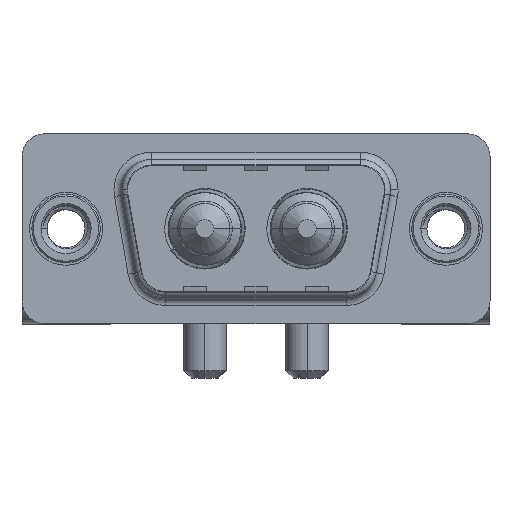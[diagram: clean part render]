
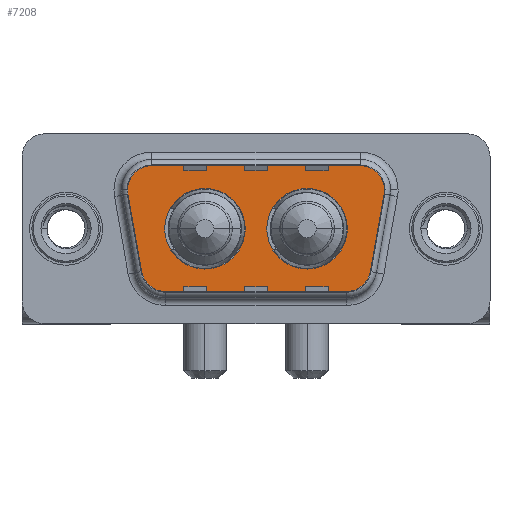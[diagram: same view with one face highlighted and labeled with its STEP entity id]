
A CAD part, top view. The second image highlights one B-rep face of the part: STEP entity #7208.
In plain terms, the highlighted planar face has unit normal (0, 0, 1).
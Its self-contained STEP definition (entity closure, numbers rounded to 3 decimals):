
#143 = CARTESIAN_POINT ( 'NONE',  ( 11.79, 0., 0. ) ) ;
#180 = VERTEX_POINT ( 'NONE', #11453 ) ;
#261 = CARTESIAN_POINT ( 'NONE',  ( 19.564, 2.9, 0. ) ) ;
#269 = EDGE_CURVE ( 'NONE', #180, #8889, #14029, .T. ) ;
#319 = EDGE_CURVE ( 'NONE', #8889, #8603, #11657, .T. ) ;
#706 = DIRECTION ( 'NONE',  ( 0., 0., 1. ) ) ;
#756 = CIRCLE ( 'NONE', #9415, 2. ) ;
#801 = CIRCLE ( 'NONE', #8774, 2.65 ) ;
#992 = CARTESIAN_POINT ( 'NONE',  ( 4.489, -3.247, 0. ) ) ;
#1006 = EDGE_CURVE ( 'NONE', #6856, #180, #7688, .T. ) ;
#1249 = CIRCLE ( 'NONE', #12812, 2.65 ) ;
#1399 = ORIENTED_EDGE ( 'NONE', *, *, #6689, .T. ) ;
#1654 = DIRECTION ( 'NONE',  ( -1., 0., 0. ) ) ;
#1833 = CARTESIAN_POINT ( 'NONE',  ( 3.466, 2.553, 0. ) ) ;
#1867 = DIRECTION ( 'NONE',  ( 0., 0., 1. ) ) ;
#1878 = CARTESIAN_POINT ( 'NONE',  ( 9.14, 0., 0. ) ) ;
#1929 = CARTESIAN_POINT ( 'NONE',  ( 21.534, 2.553, 0. ) ) ;
#1938 = CARTESIAN_POINT ( 'NONE',  ( 3.466, 2.553, 0. ) ) ;
#1943 = AXIS2_PLACEMENT_3D ( 'NONE', #5372, #4238, #2030 ) ;
#1968 = VERTEX_POINT ( 'NONE', #12082 ) ;
#2030 = DIRECTION ( 'NONE',  ( -1., 0., 0. ) ) ;
#2038 = CARTESIAN_POINT ( 'NONE',  ( 6.459, -4.9, 0. ) ) ;
#2361 = FACE_BOUND ( 'NONE', #6490, .T. ) ;
#2383 = AXIS2_PLACEMENT_3D ( 'NONE', #10458, #706, #2593 ) ;
#2424 = CARTESIAN_POINT ( 'NONE',  ( 5.436, 4.9, 0. ) ) ;
#2593 = DIRECTION ( 'NONE',  ( 1., 0., 0. ) ) ;
#2623 = CIRCLE ( 'NONE', #2383, 2.65 ) ;
#2870 = CARTESIAN_POINT ( 'NONE',  ( 6.459, -2.9, 0. ) ) ;
#3503 = CIRCLE ( 'NONE', #10978, 2. ) ;
#3579 = ORIENTED_EDGE ( 'NONE', *, *, #5162, .F. ) ;
#3752 = VERTEX_POINT ( 'NONE', #8855 ) ;
#4012 = EDGE_CURVE ( 'NONE', #6295, #6856, #756, .T. ) ;
#4131 = CARTESIAN_POINT ( 'NONE',  ( 20.511, -3.247, 0. ) ) ;
#4238 = DIRECTION ( 'NONE',  ( 0., 0., 1. ) ) ;
#4376 = CARTESIAN_POINT ( 'NONE',  ( 15.86, 0., 0. ) ) ;
#4553 = DIRECTION ( 'NONE',  ( -1., 0., 0. ) ) ;
#4625 = DIRECTION ( 'NONE',  ( 0., 0., 1. ) ) ;
#4734 = ORIENTED_EDGE ( 'NONE', *, *, #7578, .T. ) ;
#4845 = DIRECTION ( 'NONE',  ( 1., 0., 0. ) ) ;
#4931 = VERTEX_POINT ( 'NONE', #143 ) ;
#4943 = DIRECTION ( 'NONE',  ( 1., 0., 0. ) ) ;
#4959 = EDGE_LOOP ( 'NONE', ( #7784, #9993, #7604, #11183, #7877, #7526, #7380, #1399, #4734 ) ) ;
#5151 = DIRECTION ( 'NONE',  ( 1., 0., 0. ) ) ;
#5162 = EDGE_CURVE ( 'NONE', #3752, #4931, #2623, .T. ) ;
#5188 = VECTOR ( 'NONE', #4553, 1000. ) ;
#5372 = CARTESIAN_POINT ( 'NONE',  ( 19.564, 2.9, 0. ) ) ;
#5571 = EDGE_CURVE ( 'NONE', #11025, #5751, #6271, .T. ) ;
#5576 = VECTOR ( 'NONE', #13032, 1000. ) ;
#5708 = PLANE ( 'NONE',  #8068 ) ;
#5751 = VERTEX_POINT ( 'NONE', #10174 ) ;
#6210 = CARTESIAN_POINT ( 'NONE',  ( 13.21, 0., 0. ) ) ;
#6255 = EDGE_CURVE ( 'NONE', #4931, #3752, #6904, .T. ) ;
#6259 = CIRCLE ( 'NONE', #1943, 2. ) ;
#6271 = LINE ( 'NONE', #1929, #12535 ) ;
#6281 = DIRECTION ( 'NONE',  ( 0.174, -0.985, 0. ) ) ;
#6295 = VERTEX_POINT ( 'NONE', #8364 ) ;
#6349 = DIRECTION ( 'NONE',  ( 0., 0., 1. ) ) ;
#6490 = EDGE_LOOP ( 'NONE', ( #9996, #9714 ) ) ;
#6689 = EDGE_CURVE ( 'NONE', #8603, #8436, #3503, .T. ) ;
#6693 = FACE_BOUND ( 'NONE', #9036, .T. ) ;
#6771 = FACE_OUTER_BOUND ( 'NONE', #4959, .T. ) ;
#6856 = VERTEX_POINT ( 'NONE', #9342 ) ;
#6904 = CIRCLE ( 'NONE', #7358, 2.65 ) ;
#7208 = ADVANCED_FACE ( 'NONE', ( #2361, #6693, #6771 ), #5708, .T. ) ;
#7216 = EDGE_CURVE ( 'NONE', #1968, #11025, #10994, .T. ) ;
#7358 = AXIS2_PLACEMENT_3D ( 'NONE', #1878, #11670, #9429 ) ;
#7380 = ORIENTED_EDGE ( 'NONE', *, *, #319, .T. ) ;
#7526 = ORIENTED_EDGE ( 'NONE', *, *, #269, .T. ) ;
#7578 = EDGE_CURVE ( 'NONE', #8436, #1968, #10764, .T. ) ;
#7604 = ORIENTED_EDGE ( 'NONE', *, *, #8251, .T. ) ;
#7688 = LINE ( 'NONE', #2424, #5188 ) ;
#7784 = ORIENTED_EDGE ( 'NONE', *, *, #7216, .T. ) ;
#7877 = ORIENTED_EDGE ( 'NONE', *, *, #1006, .T. ) ;
#7939 = AXIS2_PLACEMENT_3D ( 'NONE', #8217, #1867, #4943 ) ;
#8068 = AXIS2_PLACEMENT_3D ( 'NONE', #10043, #13501, #4845 ) ;
#8105 = EDGE_CURVE ( 'NONE', #11201, #13163, #1249, .T. ) ;
#8217 = CARTESIAN_POINT ( 'NONE',  ( 5.436, 2.9, 0. ) ) ;
#8251 = EDGE_CURVE ( 'NONE', #5751, #6295, #6259, .T. ) ;
#8364 = CARTESIAN_POINT ( 'NONE',  ( 21.564, 2.9, 0. ) ) ;
#8413 = DIRECTION ( 'NONE',  ( 0., 0., 1. ) ) ;
#8436 = VERTEX_POINT ( 'NONE', #10540 ) ;
#8602 = EDGE_CURVE ( 'NONE', #13163, #11201, #801, .T. ) ;
#8603 = VERTEX_POINT ( 'NONE', #992 ) ;
#8774 = AXIS2_PLACEMENT_3D ( 'NONE', #12860, #6349, #5151 ) ;
#8855 = CARTESIAN_POINT ( 'NONE',  ( 6.49, 0., 0. ) ) ;
#8889 = VERTEX_POINT ( 'NONE', #1833 ) ;
#8972 = DIRECTION ( 'NONE',  ( -1., 0., 0. ) ) ;
#9036 = EDGE_LOOP ( 'NONE', ( #11649, #3579 ) ) ;
#9196 = CARTESIAN_POINT ( 'NONE',  ( 18.541, -2.9, 0. ) ) ;
#9342 = CARTESIAN_POINT ( 'NONE',  ( 19.564, 4.9, 0. ) ) ;
#9415 = AXIS2_PLACEMENT_3D ( 'NONE', #261, #4625, #8972 ) ;
#9429 = DIRECTION ( 'NONE',  ( 1., 0., 0. ) ) ;
#9714 = ORIENTED_EDGE ( 'NONE', *, *, #8602, .F. ) ;
#9849 = DIRECTION ( 'NONE',  ( 1., 0., 0. ) ) ;
#9993 = ORIENTED_EDGE ( 'NONE', *, *, #5571, .T. ) ;
#9996 = ORIENTED_EDGE ( 'NONE', *, *, #8105, .F. ) ;
#10043 = CARTESIAN_POINT ( 'NONE',  ( 18.541, -2.9, 0. ) ) ;
#10174 = CARTESIAN_POINT ( 'NONE',  ( 21.534, 2.553, 0. ) ) ;
#10247 = DIRECTION ( 'NONE',  ( 0., 0., 1. ) ) ;
#10458 = CARTESIAN_POINT ( 'NONE',  ( 9.14, 0., 0. ) ) ;
#10540 = CARTESIAN_POINT ( 'NONE',  ( 6.459, -4.9, 0. ) ) ;
#10755 = AXIS2_PLACEMENT_3D ( 'NONE', #9196, #10247, #11366 ) ;
#10764 = LINE ( 'NONE', #2038, #5576 ) ;
#10978 = AXIS2_PLACEMENT_3D ( 'NONE', #2870, #8413, #1654 ) ;
#10994 = CIRCLE ( 'NONE', #10755, 2. ) ;
#11025 = VERTEX_POINT ( 'NONE', #4131 ) ;
#11183 = ORIENTED_EDGE ( 'NONE', *, *, #4012, .T. ) ;
#11201 = VERTEX_POINT ( 'NONE', #12069 ) ;
#11366 = DIRECTION ( 'NONE',  ( 1., 0., 0. ) ) ;
#11453 = CARTESIAN_POINT ( 'NONE',  ( 5.436, 4.9, 0. ) ) ;
#11649 = ORIENTED_EDGE ( 'NONE', *, *, #6255, .F. ) ;
#11657 = LINE ( 'NONE', #1938, #13340 ) ;
#11670 = DIRECTION ( 'NONE',  ( 0., 0., 1. ) ) ;
#12069 = CARTESIAN_POINT ( 'NONE',  ( 18.51, 0., 0. ) ) ;
#12082 = CARTESIAN_POINT ( 'NONE',  ( 18.541, -4.9, 0. ) ) ;
#12535 = VECTOR ( 'NONE', #13992, 1000. ) ;
#12804 = DIRECTION ( 'NONE',  ( 0., 0., 1. ) ) ;
#12812 = AXIS2_PLACEMENT_3D ( 'NONE', #4376, #12804, #9849 ) ;
#12860 = CARTESIAN_POINT ( 'NONE',  ( 15.86, 0., 0. ) ) ;
#13032 = DIRECTION ( 'NONE',  ( 1., 0., 0. ) ) ;
#13163 = VERTEX_POINT ( 'NONE', #6210 ) ;
#13340 = VECTOR ( 'NONE', #6281, 1000. ) ;
#13501 = DIRECTION ( 'NONE',  ( 0., 0., 1. ) ) ;
#13992 = DIRECTION ( 'NONE',  ( 0.174, 0.985, 0. ) ) ;
#14029 = CIRCLE ( 'NONE', #7939, 2. ) ;
